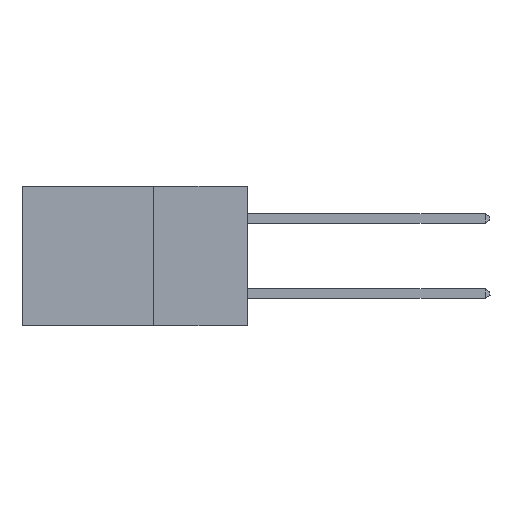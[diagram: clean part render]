
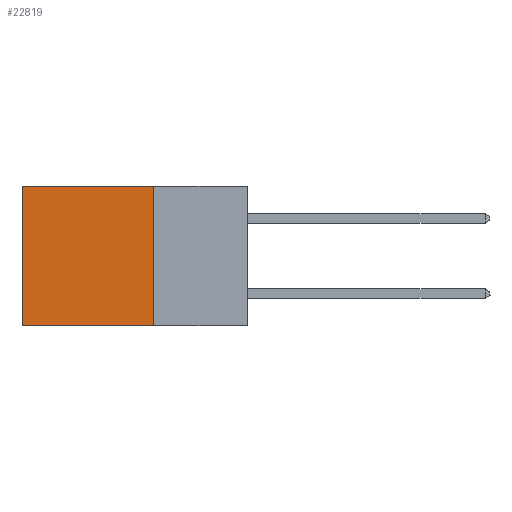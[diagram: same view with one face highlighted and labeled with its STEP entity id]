
A CAD part, left-side view. The second image highlights one B-rep face of the part: STEP entity #22819.
In plain terms, the highlighted planar face has unit normal (-1, 0, 0).
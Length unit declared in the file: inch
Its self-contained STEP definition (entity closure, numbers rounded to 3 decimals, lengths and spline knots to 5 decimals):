
#666 = EDGE_CURVE ( 'NONE', #2688, #12394, #14163, .T. ) ;
#810 = VECTOR ( 'NONE', #10723, 39.37008 ) ;
#909 = CARTESIAN_POINT ( 'NONE',  ( 0.298, 0.6, 0. ) ) ;
#1944 = VECTOR ( 'NONE', #2496, 39.37008 ) ;
#2463 = EDGE_CURVE ( 'NONE', #2515, #12394, #8037, .T. ) ;
#2462 = VECTOR ( 'NONE', #14048, 39.37008 ) ;
#2496 = DIRECTION ( 'NONE',  ( 0., 0., -1. ) ) ;
#2515 = VERTEX_POINT ( 'NONE', #7008 ) ;
#2688 = VERTEX_POINT ( 'NONE', #21782 ) ;
#3490 = CARTESIAN_POINT ( 'NONE',  ( 0.298, 0.25, 0. ) ) ;
#5351 = DIRECTION ( 'NONE',  ( 1., 0., 0. ) ) ;
#5401 = VECTOR ( 'NONE', #19543, 39.37008 ) ;
#6859 = LINE ( 'NONE', #14069, #5401 ) ;
#7008 = CARTESIAN_POINT ( 'NONE',  ( 0.298, 0.6, 0. ) ) ;
#8037 = LINE ( 'NONE', #909, #2462 ) ;
#9341 = ORIENTED_EDGE ( 'NONE', *, *, #17079, .F. ) ;
#10723 = DIRECTION ( 'NONE',  ( 0., 1., 0. ) ) ;
#11380 = VERTEX_POINT ( 'NONE', #14791 ) ;
#11483 = ORIENTED_EDGE ( 'NONE', *, *, #12620, .T. ) ;
#12394 = VERTEX_POINT ( 'NONE', #19975 ) ;
#12620 = EDGE_CURVE ( 'NONE', #11380, #2515, #6859, .T. ) ;
#12759 = EDGE_LOOP ( 'NONE', ( #20349, #21504, #9341, #11483 ) ) ;
#13631 = CARTESIAN_POINT ( 'NONE',  ( 0.298, 0.25, 0. ) ) ;
#13678 = AXIS2_PLACEMENT_3D ( 'NONE', #3490, #5351, #20205 ) ;
#14048 = DIRECTION ( 'NONE',  ( 0., 0., -1. ) ) ;
#14069 = CARTESIAN_POINT ( 'NONE',  ( 0.298, 0.25, 0. ) ) ;
#14163 = LINE ( 'NONE', #19781, #810 ) ;
#14791 = CARTESIAN_POINT ( 'NONE',  ( 0.298, 0.25, 0. ) ) ;
#15884 = LINE ( 'NONE', #13631, #1944 ) ;
#17079 = EDGE_CURVE ( 'NONE', #11380, #2688, #15884, .T. ) ;
#19543 = DIRECTION ( 'NONE',  ( 0., 1., 0. ) ) ;
#19781 = CARTESIAN_POINT ( 'NONE',  ( 0.298, 0.25, -0.37 ) ) ;
#19975 = CARTESIAN_POINT ( 'NONE',  ( 0.298, 0.6, -0.37 ) ) ;
#20205 = DIRECTION ( 'NONE',  ( 0., 0., -1. ) ) ;
#20349 = ORIENTED_EDGE ( 'NONE', *, *, #2463, .T. ) ;
#21015 = FACE_OUTER_BOUND ( 'NONE', #12759, .T. ) ;
#21504 = ORIENTED_EDGE ( 'NONE', *, *, #666, .F. ) ;
#21782 = CARTESIAN_POINT ( 'NONE',  ( 0.298, 0.25, -0.37 ) ) ;
#22019 = PLANE ( 'NONE',  #13678 ) ;
#22819 = ADVANCED_FACE ( 'NONE', ( #21015 ), #22019, .F. ) ;
